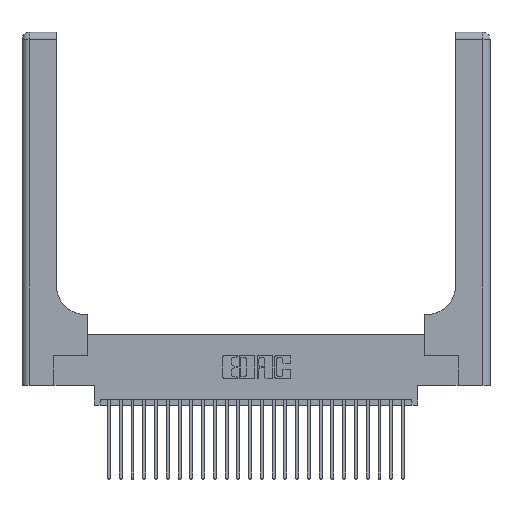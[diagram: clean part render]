
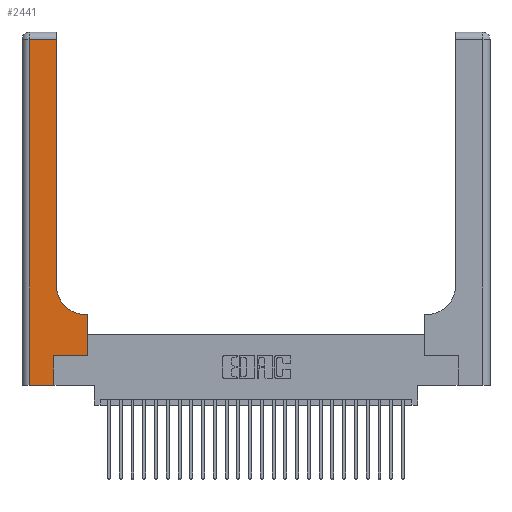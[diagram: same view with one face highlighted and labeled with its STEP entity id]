
A CAD part, top view. The second image highlights one B-rep face of the part: STEP entity #2441.
In plain terms, the highlighted planar face has unit normal (0, 0, 1).
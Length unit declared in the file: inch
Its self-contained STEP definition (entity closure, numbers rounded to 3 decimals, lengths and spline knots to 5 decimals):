
#2426 = CARTESIAN_POINT ( 'NONE',  ( 0.5585, 0.6, 0.37 ) ) ;
#2441 = ADVANCED_FACE ( 'NONE', ( #12218 ), #6539, .F. ) ;
#2715 = VERTEX_POINT ( 'NONE', #6368 ) ;
#2927 = CARTESIAN_POINT ( 'NONE',  ( 0.2915, 0.6, 0.37 ) ) ;
#3051 = LINE ( 'NONE', #9585, #13478 ) ;
#3371 = ORIENTED_EDGE ( 'NONE', *, *, #14720, .T. ) ;
#3888 = VERTEX_POINT ( 'NONE', #12603 ) ;
#4159 = DIRECTION ( 'NONE',  ( -1., 0., 0. ) ) ;
#4463 = VECTOR ( 'NONE', #19762, 39.37008 ) ;
#4920 = VECTOR ( 'NONE', #4159, 39.37008 ) ;
#5088 = DIRECTION ( 'NONE',  ( 0., 1., 0. ) ) ;
#6122 = DIRECTION ( 'NONE',  ( 1., 0., 0. ) ) ;
#6368 = CARTESIAN_POINT ( 'NONE',  ( 0.269, 0., 0.37 ) ) ;
#6539 = PLANE ( 'NONE',  #14376 ) ;
#6913 = CARTESIAN_POINT ( 'NONE',  ( 0.5415, 0.6, 0.37 ) ) ;
#7299 = VECTOR ( 'NONE', #9472, 39.37008 ) ;
#7449 = EDGE_CURVE ( 'NONE', #8628, #24311, #27463, .T. ) ;
#7732 = EDGE_CURVE ( 'NONE', #2715, #24866, #3051, .T. ) ;
#7976 = CARTESIAN_POINT ( 'NONE',  ( 0.06, 3., 0.37 ) ) ;
#8220 = CARTESIAN_POINT ( 'NONE',  ( 0., 2.94, 0.37 ) ) ;
#8258 = CARTESIAN_POINT ( 'NONE',  ( 0.269, 0.25, 0.37 ) ) ;
#8628 = VERTEX_POINT ( 'NONE', #6913 ) ;
#8851 = LINE ( 'NONE', #17411, #4463 ) ;
#8980 = CARTESIAN_POINT ( 'NONE',  ( 0., 3., 0.37 ) ) ;
#8997 = VECTOR ( 'NONE', #9531, 39.37008 ) ;
#9472 = DIRECTION ( 'NONE',  ( -1., 0., 0. ) ) ;
#9531 = DIRECTION ( 'NONE',  ( 0., 1., 0. ) ) ;
#9585 = CARTESIAN_POINT ( 'NONE',  ( 0.269, 0., 0.37 ) ) ;
#10093 = ORIENTED_EDGE ( 'NONE', *, *, #14303, .T. ) ;
#10550 = EDGE_LOOP ( 'NONE', ( #24099, #14296, #21217, #3371, #21724, #10093, #21737, #16814, #21157 ) ) ;
#10705 = DIRECTION ( 'NONE',  ( 0., 0., -1. ) ) ;
#11750 = VECTOR ( 'NONE', #12309, 39.37008 ) ;
#12205 = EDGE_CURVE ( 'NONE', #18008, #8628, #20766, .T. ) ;
#12218 = FACE_OUTER_BOUND ( 'NONE', #10550, .T. ) ;
#12284 = DIRECTION ( 'NONE',  ( 1., 0., 0. ) ) ;
#12309 = DIRECTION ( 'NONE',  ( 0., -1., 0. ) ) ;
#12603 = CARTESIAN_POINT ( 'NONE',  ( 0.2915, 2.94, 0.37 ) ) ;
#13467 = DIRECTION ( 'NONE',  ( 0., 0., -1. ) ) ;
#13478 = VECTOR ( 'NONE', #5088, 39.37008 ) ;
#14107 = EDGE_CURVE ( 'NONE', #16357, #17882, #16174, .T. ) ;
#14296 = ORIENTED_EDGE ( 'NONE', *, *, #20163, .T. ) ;
#14303 = EDGE_CURVE ( 'NONE', #24866, #16557, #17664, .T. ) ;
#14354 = CARTESIAN_POINT ( 'NONE',  ( 0.5585, 0.25, 0.37 ) ) ;
#14376 = AXIS2_PLACEMENT_3D ( 'NONE', #8980, #13467, #24391 ) ;
#14496 = CARTESIAN_POINT ( 'NONE',  ( 0.269, 0.25, 0.37 ) ) ;
#14720 = EDGE_CURVE ( 'NONE', #17882, #2715, #15292, .T. ) ;
#15292 = LINE ( 'NONE', #27604, #22700 ) ;
#15521 = EDGE_CURVE ( 'NONE', #16557, #18008, #8851, .T. ) ;
#15535 = AXIS2_PLACEMENT_3D ( 'NONE', #19196, #10705, #6122 ) ;
#16174 = LINE ( 'NONE', #7976, #11750 ) ;
#16357 = VERTEX_POINT ( 'NONE', #22076 ) ;
#16557 = VERTEX_POINT ( 'NONE', #14354 ) ;
#16814 = ORIENTED_EDGE ( 'NONE', *, *, #12205, .T. ) ;
#17266 = CARTESIAN_POINT ( 'NONE',  ( 0.06, 0., 0.37 ) ) ;
#17411 = CARTESIAN_POINT ( 'NONE',  ( 0.5585, 0.25, 0.37 ) ) ;
#17664 = LINE ( 'NONE', #8258, #19021 ) ;
#17882 = VERTEX_POINT ( 'NONE', #17266 ) ;
#18008 = VERTEX_POINT ( 'NONE', #2426 ) ;
#18213 = CARTESIAN_POINT ( 'NONE',  ( 0.2915, 3., 0.37 ) ) ;
#19021 = VECTOR ( 'NONE', #25465, 39.37008 ) ;
#19196 = CARTESIAN_POINT ( 'NONE',  ( 0.5415, 0.85, 0.37 ) ) ;
#19468 = EDGE_CURVE ( 'NONE', #24311, #3888, #20461, .T. ) ;
#19762 = DIRECTION ( 'NONE',  ( 0., 1., 0. ) ) ;
#20065 = LINE ( 'NONE', #8220, #4920 ) ;
#20163 = EDGE_CURVE ( 'NONE', #3888, #16357, #20065, .T. ) ;
#20461 = LINE ( 'NONE', #18213, #8997 ) ;
#20766 = LINE ( 'NONE', #2927, #7299 ) ;
#21157 = ORIENTED_EDGE ( 'NONE', *, *, #7449, .T. ) ;
#21217 = ORIENTED_EDGE ( 'NONE', *, *, #14107, .T. ) ;
#21724 = ORIENTED_EDGE ( 'NONE', *, *, #7732, .T. ) ;
#21737 = ORIENTED_EDGE ( 'NONE', *, *, #15521, .T. ) ;
#22076 = CARTESIAN_POINT ( 'NONE',  ( 0.06, 2.94, 0.37 ) ) ;
#22700 = VECTOR ( 'NONE', #12284, 39.37008 ) ;
#24099 = ORIENTED_EDGE ( 'NONE', *, *, #19468, .T. ) ;
#24311 = VERTEX_POINT ( 'NONE', #26460 ) ;
#24391 = DIRECTION ( 'NONE',  ( -1., 0., 0. ) ) ;
#24866 = VERTEX_POINT ( 'NONE', #14496 ) ;
#25465 = DIRECTION ( 'NONE',  ( 1., 0., 0. ) ) ;
#26460 = CARTESIAN_POINT ( 'NONE',  ( 0.2915, 0.85, 0.37 ) ) ;
#27463 = CIRCLE ( 'NONE', #15535, 0.25 ) ;
#27604 = CARTESIAN_POINT ( 'NONE',  ( 0., 0., 0.37 ) ) ;
